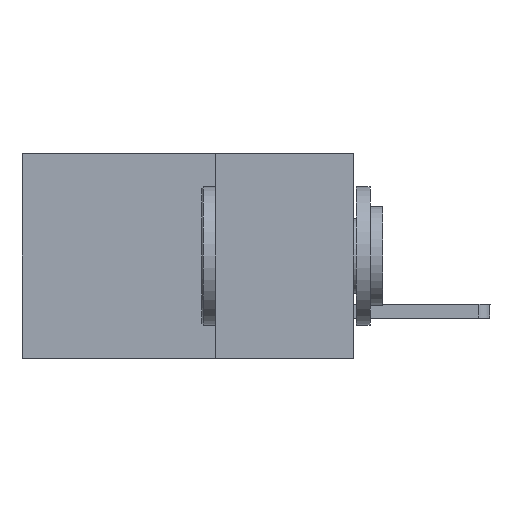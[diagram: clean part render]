
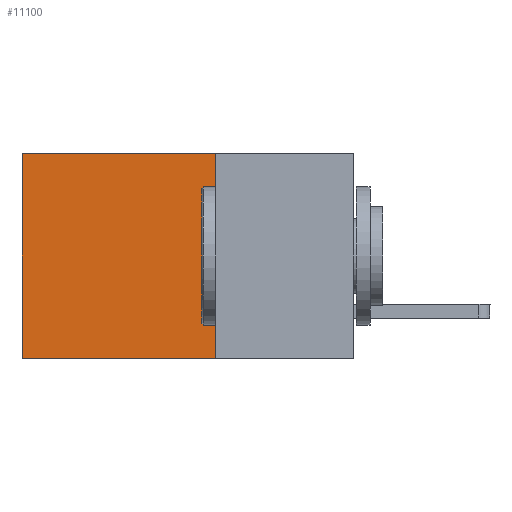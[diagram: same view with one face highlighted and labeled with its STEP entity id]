
A CAD part, left-side view. The second image highlights one B-rep face of the part: STEP entity #11100.
In plain terms, the highlighted planar face has unit normal (-1, 0, 0).
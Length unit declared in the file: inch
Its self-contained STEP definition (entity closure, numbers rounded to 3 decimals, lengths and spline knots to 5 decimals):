
#393 = EDGE_CURVE ( 'NONE', #3848, #1125, #8925, .T. ) ;
#626 = DIRECTION ( 'NONE',  ( 0., 1., 0. ) ) ;
#691 = VERTEX_POINT ( 'NONE', #2554 ) ;
#1125 = VERTEX_POINT ( 'NONE', #8943 ) ;
#1266 = VECTOR ( 'NONE', #3570, 39.37008 ) ;
#1428 = CARTESIAN_POINT ( 'NONE',  ( 0.2875, 0.25, 0. ) ) ;
#2066 = DIRECTION ( 'NONE',  ( 1., 0., 0. ) ) ;
#2095 = LINE ( 'NONE', #5873, #8059 ) ;
#2444 = ORIENTED_EDGE ( 'NONE', *, *, #3549, .T. ) ;
#2548 = VERTEX_POINT ( 'NONE', #11238 ) ;
#2554 = CARTESIAN_POINT ( 'NONE',  ( 0.2875, 0.6, 0. ) ) ;
#3549 = EDGE_CURVE ( 'NONE', #3848, #691, #6557, .T. ) ;
#3570 = DIRECTION ( 'NONE',  ( 0., 0., -1. ) ) ;
#3848 = VERTEX_POINT ( 'NONE', #4471 ) ;
#3851 = DIRECTION ( 'NONE',  ( 0., 0., -1. ) ) ;
#4430 = LINE ( 'NONE', #7898, #1266 ) ;
#4471 = CARTESIAN_POINT ( 'NONE',  ( 0.2875, 0.25, 0. ) ) ;
#4896 = EDGE_CURVE ( 'NONE', #691, #2548, #4430, .T. ) ;
#5711 = DIRECTION ( 'NONE',  ( 0., 1., 0. ) ) ;
#5745 = ORIENTED_EDGE ( 'NONE', *, *, #4896, .T. ) ;
#5873 = CARTESIAN_POINT ( 'NONE',  ( 0.2875, 0.25, -0.37 ) ) ;
#6557 = LINE ( 'NONE', #7085, #9836 ) ;
#6575 = CARTESIAN_POINT ( 'NONE',  ( 0.2875, 0.25, 0. ) ) ;
#6897 = ORIENTED_EDGE ( 'NONE', *, *, #10731, .F. ) ;
#7041 = FACE_OUTER_BOUND ( 'NONE', #11559, .T. ) ;
#7085 = CARTESIAN_POINT ( 'NONE',  ( 0.2875, 0.25, 0. ) ) ;
#7430 = ORIENTED_EDGE ( 'NONE', *, *, #393, .F. ) ;
#7898 = CARTESIAN_POINT ( 'NONE',  ( 0.2875, 0.6, 0. ) ) ;
#8059 = VECTOR ( 'NONE', #5711, 39.37008 ) ;
#8748 = DIRECTION ( 'NONE',  ( 0., 0., -1. ) ) ;
#8925 = LINE ( 'NONE', #1428, #11524 ) ;
#8943 = CARTESIAN_POINT ( 'NONE',  ( 0.2875, 0.25, -0.37 ) ) ;
#9836 = VECTOR ( 'NONE', #626, 39.37008 ) ;
#10172 = PLANE ( 'NONE',  #11360 ) ;
#10731 = EDGE_CURVE ( 'NONE', #1125, #2548, #2095, .T. ) ;
#11100 = ADVANCED_FACE ( 'NONE', ( #7041 ), #10172, .F. ) ;
#11238 = CARTESIAN_POINT ( 'NONE',  ( 0.2875, 0.6, -0.37 ) ) ;
#11360 = AXIS2_PLACEMENT_3D ( 'NONE', #6575, #2066, #3851 ) ;
#11524 = VECTOR ( 'NONE', #8748, 39.37008 ) ;
#11559 = EDGE_LOOP ( 'NONE', ( #5745, #6897, #7430, #2444 ) ) ;
